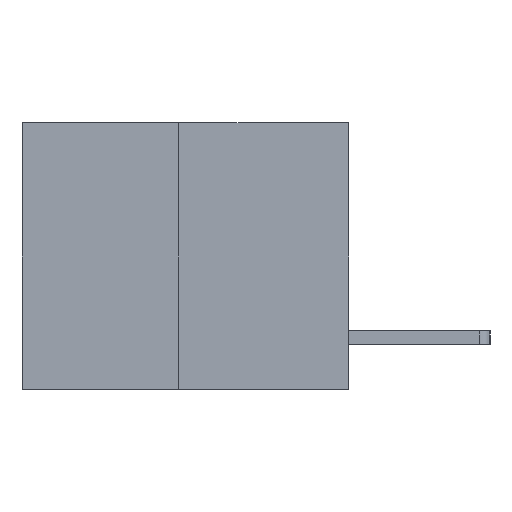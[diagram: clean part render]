
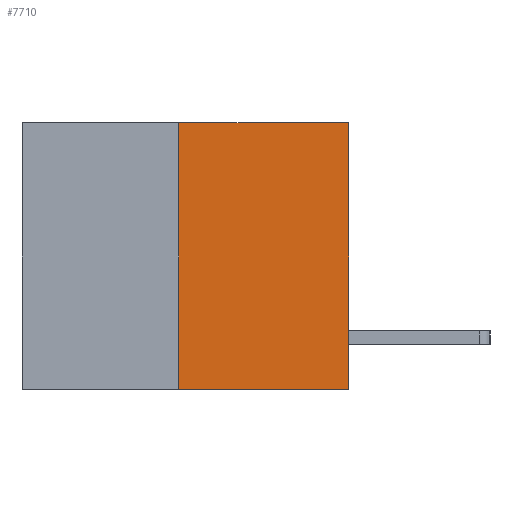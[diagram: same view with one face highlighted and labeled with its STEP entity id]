
A CAD part, left-side view. The second image highlights one B-rep face of the part: STEP entity #7710.
In plain terms, the highlighted planar face has unit normal (-1, 0, 0).
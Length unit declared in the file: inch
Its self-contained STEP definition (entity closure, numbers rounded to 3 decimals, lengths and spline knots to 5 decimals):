
#63 = EDGE_CURVE ( 'NONE', #7781, #1548, #5271, .T. ) ;
#543 = CARTESIAN_POINT ( 'NONE',  ( 0., 0.6, 0. ) ) ;
#899 = CARTESIAN_POINT ( 'NONE',  ( 0., 0.312, 0. ) ) ;
#1446 = ORIENTED_EDGE ( 'NONE', *, *, #2412, .T. ) ;
#1548 = VERTEX_POINT ( 'NONE', #899 ) ;
#1722 = DIRECTION ( 'NONE',  ( 0., -1., 0. ) ) ;
#1793 = ORIENTED_EDGE ( 'NONE', *, *, #5811, .T. ) ;
#1927 = DIRECTION ( 'NONE',  ( 1., 0., 0. ) ) ;
#2412 = EDGE_CURVE ( 'NONE', #7781, #11807, #9733, .T. ) ;
#2552 = CARTESIAN_POINT ( 'NONE',  ( 0., 0., 0. ) ) ;
#2887 = LINE ( 'NONE', #543, #3347 ) ;
#2888 = VECTOR ( 'NONE', #6360, 39.37008 ) ;
#3347 = VECTOR ( 'NONE', #7555, 39.37008 ) ;
#3553 = VECTOR ( 'NONE', #5173, 39.37008 ) ;
#3894 = CARTESIAN_POINT ( 'NONE',  ( 0., 0., 0. ) ) ;
#3952 = EDGE_LOOP ( 'NONE', ( #7452, #1446, #1793, #4988 ) ) ;
#4098 = CARTESIAN_POINT ( 'NONE',  ( 0., 0., -0.49 ) ) ;
#4988 = ORIENTED_EDGE ( 'NONE', *, *, #5185, .F. ) ;
#5173 = DIRECTION ( 'NONE',  ( 0., 0., 1. ) ) ;
#5185 = EDGE_CURVE ( 'NONE', #1548, #9039, #2887, .T. ) ;
#5257 = VECTOR ( 'NONE', #1722, 39.37008 ) ;
#5271 = LINE ( 'NONE', #9105, #3553 ) ;
#5525 = LINE ( 'NONE', #2552, #2888 ) ;
#5811 = EDGE_CURVE ( 'NONE', #11807, #9039, #5525, .T. ) ;
#5830 = PLANE ( 'NONE',  #6304 ) ;
#6304 = AXIS2_PLACEMENT_3D ( 'NONE', #8829, #1927, #11745 ) ;
#6360 = DIRECTION ( 'NONE',  ( 0., 0., 1. ) ) ;
#6705 = CARTESIAN_POINT ( 'NONE',  ( 0., 0.6, -0.49 ) ) ;
#7452 = ORIENTED_EDGE ( 'NONE', *, *, #63, .F. ) ;
#7555 = DIRECTION ( 'NONE',  ( 0., -1., 0. ) ) ;
#7710 = ADVANCED_FACE ( 'NONE', ( #8417 ), #5830, .F. ) ;
#7781 = VERTEX_POINT ( 'NONE', #8746 ) ;
#8417 = FACE_OUTER_BOUND ( 'NONE', #3952, .T. ) ;
#8746 = CARTESIAN_POINT ( 'NONE',  ( 0., 0.312, -0.49 ) ) ;
#8829 = CARTESIAN_POINT ( 'NONE',  ( 0., 0.6, 0. ) ) ;
#9039 = VERTEX_POINT ( 'NONE', #3894 ) ;
#9105 = CARTESIAN_POINT ( 'NONE',  ( 0., 0.312, -0.49 ) ) ;
#9733 = LINE ( 'NONE', #6705, #5257 ) ;
#11745 = DIRECTION ( 'NONE',  ( 0., 0., -1. ) ) ;
#11807 = VERTEX_POINT ( 'NONE', #4098 ) ;
